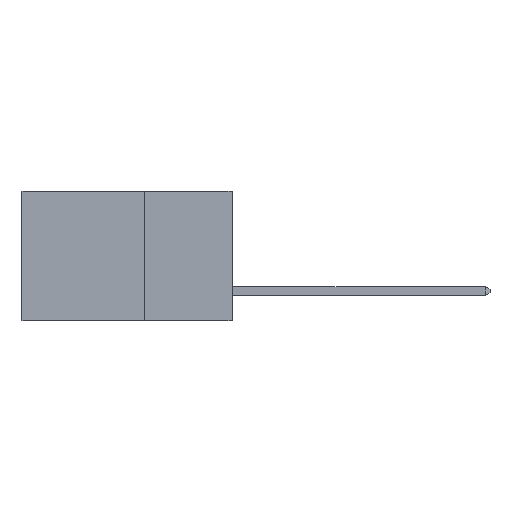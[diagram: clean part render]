
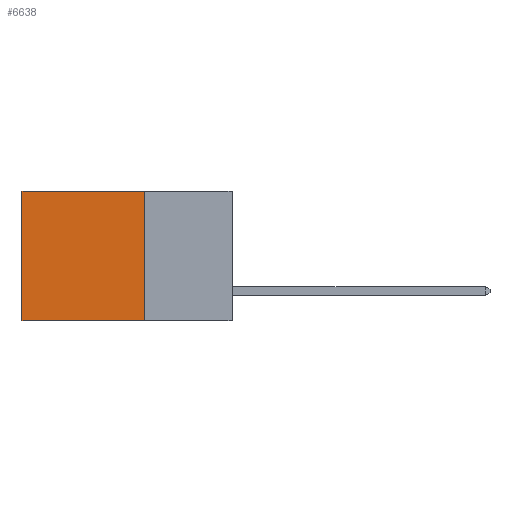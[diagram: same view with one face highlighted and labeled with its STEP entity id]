
A CAD part, left-side view. The second image highlights one B-rep face of the part: STEP entity #6638.
In plain terms, the highlighted planar face has unit normal (-1, 0, 0).
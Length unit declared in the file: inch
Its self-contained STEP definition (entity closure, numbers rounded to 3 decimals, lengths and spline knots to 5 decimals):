
#36 = CARTESIAN_POINT ( 'NONE',  ( 0.2875, 0.6, -0.37 ) ) ;
#737 = VECTOR ( 'NONE', #6459, 39.37008 ) ;
#1150 = VECTOR ( 'NONE', #15202, 39.37008 ) ;
#1217 = ORIENTED_EDGE ( 'NONE', *, *, #13803, .T. ) ;
#1377 = VERTEX_POINT ( 'NONE', #3150 ) ;
#2940 = AXIS2_PLACEMENT_3D ( 'NONE', #14218, #5685, #15509 ) ;
#2957 = LINE ( 'NONE', #6366, #9939 ) ;
#3150 = CARTESIAN_POINT ( 'NONE',  ( 0.2875, 0.25, 0. ) ) ;
#3250 = VERTEX_POINT ( 'NONE', #36 ) ;
#3284 = VERTEX_POINT ( 'NONE', #3460 ) ;
#3342 = EDGE_CURVE ( 'NONE', #7990, #3250, #8717, .T. ) ;
#3460 = CARTESIAN_POINT ( 'NONE',  ( 0.2875, 0.25, -0.37 ) ) ;
#4345 = EDGE_CURVE ( 'NONE', #3284, #3250, #5229, .T. ) ;
#4872 = DIRECTION ( 'NONE',  ( 0., 0., -1. ) ) ;
#5229 = LINE ( 'NONE', #15292, #1150 ) ;
#5685 = DIRECTION ( 'NONE',  ( 1., 0., 0. ) ) ;
#6366 = CARTESIAN_POINT ( 'NONE',  ( 0.2875, 0.25, 0. ) ) ;
#6459 = DIRECTION ( 'NONE',  ( 0., 0., -1. ) ) ;
#6638 = ADVANCED_FACE ( 'NONE', ( #7435 ), #10014, .F. ) ;
#7171 = LINE ( 'NONE', #10347, #14258 ) ;
#7435 = FACE_OUTER_BOUND ( 'NONE', #13781, .T. ) ;
#7990 = VERTEX_POINT ( 'NONE', #10096 ) ;
#8717 = LINE ( 'NONE', #8895, #737 ) ;
#8885 = DIRECTION ( 'NONE',  ( 0., 1., 0. ) ) ;
#8895 = CARTESIAN_POINT ( 'NONE',  ( 0.2875, 0.6, 0. ) ) ;
#9939 = VECTOR ( 'NONE', #4872, 39.37008 ) ;
#10014 = PLANE ( 'NONE',  #2940 ) ;
#10096 = CARTESIAN_POINT ( 'NONE',  ( 0.2875, 0.6, 0. ) ) ;
#10347 = CARTESIAN_POINT ( 'NONE',  ( 0.2875, 0.25, 0. ) ) ;
#12704 = EDGE_CURVE ( 'NONE', #1377, #3284, #2957, .T. ) ;
#13781 = EDGE_LOOP ( 'NONE', ( #17441, #14451, #17526, #1217 ) ) ;
#13803 = EDGE_CURVE ( 'NONE', #1377, #7990, #7171, .T. ) ;
#14218 = CARTESIAN_POINT ( 'NONE',  ( 0.2875, 0.25, 0. ) ) ;
#14258 = VECTOR ( 'NONE', #8885, 39.37008 ) ;
#14451 = ORIENTED_EDGE ( 'NONE', *, *, #4345, .F. ) ;
#15202 = DIRECTION ( 'NONE',  ( 0., 1., 0. ) ) ;
#15292 = CARTESIAN_POINT ( 'NONE',  ( 0.2875, 0.25, -0.37 ) ) ;
#15509 = DIRECTION ( 'NONE',  ( 0., 0., -1. ) ) ;
#17441 = ORIENTED_EDGE ( 'NONE', *, *, #3342, .T. ) ;
#17526 = ORIENTED_EDGE ( 'NONE', *, *, #12704, .F. ) ;
